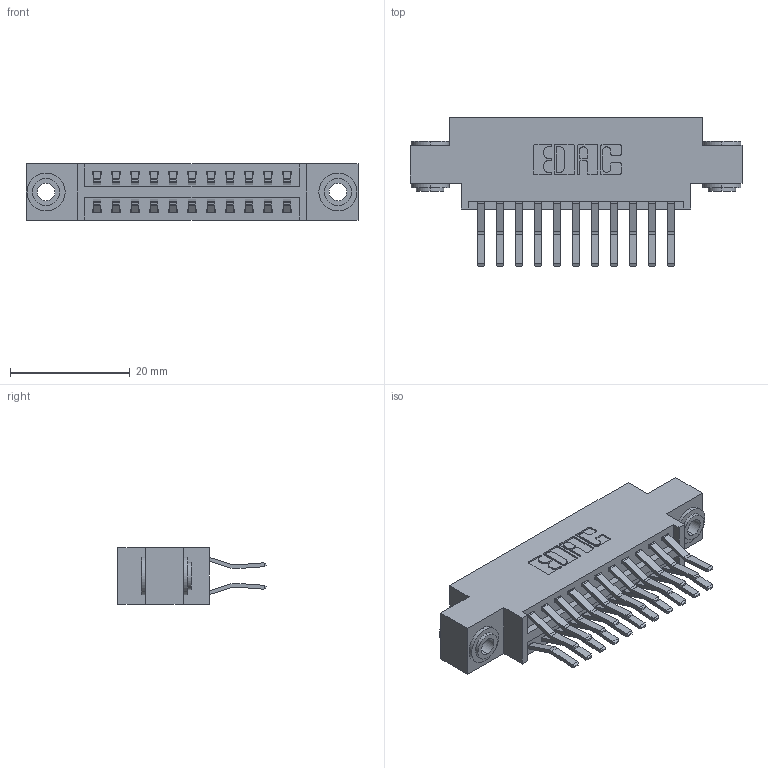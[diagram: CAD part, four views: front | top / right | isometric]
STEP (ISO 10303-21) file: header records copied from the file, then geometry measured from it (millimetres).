
FILE_DESCRIPTION (( 'STEP AP203' ), '1' );
FILE_NAME ('396-022-560-803.STEP', '2018-09-01T11:10:41', ( '' ), ( '' ), 'SwSTEP 2.0', 'SolidWorks 2016', '' );
FILE_SCHEMA (( 'CONFIG_CONTROL_DESIGN' ));
Length unit declared in the file: inch
Products named in the file (4): 346 Part_0.170 Offset - 0.156 Dia-TH; 345-292-001_560 Tail; 345-250-002_345-250-002-102; 396-022-560-803
Assembly tree (25 placements, depth 2):
  396-022-560-803
    346 Part_0.170 Offset - 0.156 Dia-TH
    345-292-001_560 Tail  x22
    345-250-002_345-250-002-102  x2
Bounding box: 55.5 x 24.78 x 9.4 mm (x, y, z)
Volume: 5180.1 mm3; surface area: 7411.6 mm2
Topology: 25 solids, 25 shells, 1352 faces, 3959 edges, 2606 vertices
Faces by surface type: plane 860, cylinder 484, cone 8
Entity records: 12222 total; most frequent: CARTESIAN_POINT 2035, ORIENTED_EDGE 1962, DIRECTION 1879, EDGE_CURVE 981, VECTOR 777, LINE 777, VERTEX_POINT 650, AXIS2_PLACEMENT_3D 551
